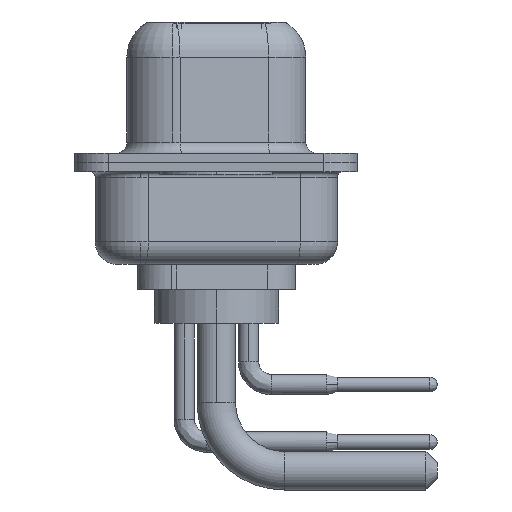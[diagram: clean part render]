
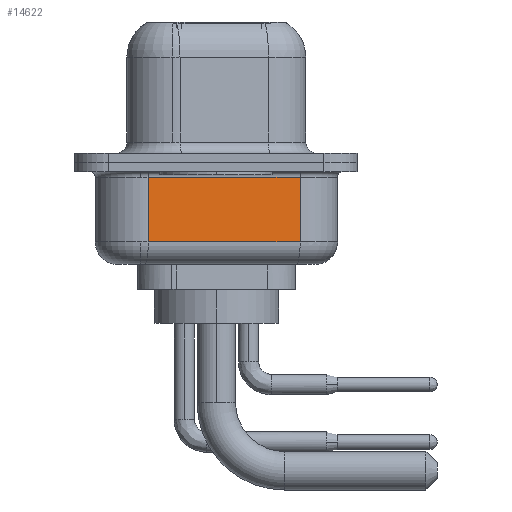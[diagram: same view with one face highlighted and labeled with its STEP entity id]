
A CAD part, left-side view. The second image highlights one B-rep face of the part: STEP entity #14622.
In plain terms, the highlighted planar face has unit normal (-0.985, -0.174, 0).
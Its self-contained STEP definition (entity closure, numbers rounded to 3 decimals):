
#284 = CARTESIAN_POINT ( 'NONE',  ( 4.062, -3.697, -4.5 ) ) ;
#936 = VERTEX_POINT ( 'NONE', #15706 ) ;
#1621 = LINE ( 'NONE', #284, #11083 ) ;
#1630 = VERTEX_POINT ( 'NONE', #12228 ) ;
#2819 = EDGE_CURVE ( 'NONE', #936, #1630, #13065, .T. ) ;
#4890 = CARTESIAN_POINT ( 'NONE',  ( 2.88, 3.003, -4.5 ) ) ;
#5376 = VECTOR ( 'NONE', #16734, 1000. ) ;
#7223 = CARTESIAN_POINT ( 'NONE',  ( 4.062, -3.697, -3.5 ) ) ;
#9784 = VERTEX_POINT ( 'NONE', #19284 ) ;
#9912 = ORIENTED_EDGE ( 'NONE', *, *, #2819, .T. ) ;
#10346 = EDGE_CURVE ( 'NONE', #9784, #1630, #15489, .T. ) ;
#10744 = DIRECTION ( 'NONE',  ( 0.985, 0.174, 0. ) ) ;
#11083 = VECTOR ( 'NONE', #15552, 1000. ) ;
#11203 = VECTOR ( 'NONE', #16923, 1000. ) ;
#12228 = CARTESIAN_POINT ( 'NONE',  ( 2.88, 3.003, -0.65 ) ) ;
#12762 = FACE_OUTER_BOUND ( 'NONE', #14419, .T. ) ;
#13065 = LINE ( 'NONE', #16023, #15784 ) ;
#14419 = EDGE_LOOP ( 'NONE', ( #16539, #15902, #16383, #9912 ) ) ;
#14622 = ADVANCED_FACE ( 'NONE', ( #12762 ), #17096, .F. ) ;
#14642 = EDGE_CURVE ( 'NONE', #15373, #936, #1621, .T. ) ;
#14664 = AXIS2_PLACEMENT_3D ( 'NONE', #4890, #10744, #17284 ) ;
#14886 = LINE ( 'NONE', #18268, #5376 ) ;
#15373 = VERTEX_POINT ( 'NONE', #7223 ) ;
#15453 = EDGE_CURVE ( 'NONE', #9784, #15373, #14886, .T. ) ;
#15489 = LINE ( 'NONE', #16714, #11203 ) ;
#15552 = DIRECTION ( 'NONE',  ( 0., 0., 1. ) ) ;
#15706 = CARTESIAN_POINT ( 'NONE',  ( 4.062, -3.697, -0.65 ) ) ;
#15784 = VECTOR ( 'NONE', #19300, 1000. ) ;
#15902 = ORIENTED_EDGE ( 'NONE', *, *, #15453, .T. ) ;
#16023 = CARTESIAN_POINT ( 'NONE',  ( 2.88, 3.003, -0.65 ) ) ;
#16383 = ORIENTED_EDGE ( 'NONE', *, *, #14642, .T. ) ;
#16539 = ORIENTED_EDGE ( 'NONE', *, *, #10346, .F. ) ;
#16714 = CARTESIAN_POINT ( 'NONE',  ( 2.88, 3.003, -4.5 ) ) ;
#16734 = DIRECTION ( 'NONE',  ( 0.174, -0.985, 0. ) ) ;
#16923 = DIRECTION ( 'NONE',  ( 0., 0., 1. ) ) ;
#17096 = PLANE ( 'NONE',  #14664 ) ;
#17284 = DIRECTION ( 'NONE',  ( -0.174, 0.985, 0. ) ) ;
#18268 = CARTESIAN_POINT ( 'NONE',  ( 2.88, 3.003, -3.5 ) ) ;
#19284 = CARTESIAN_POINT ( 'NONE',  ( 2.88, 3.003, -3.5 ) ) ;
#19300 = DIRECTION ( 'NONE',  ( -0.174, 0.985, 0. ) ) ;
